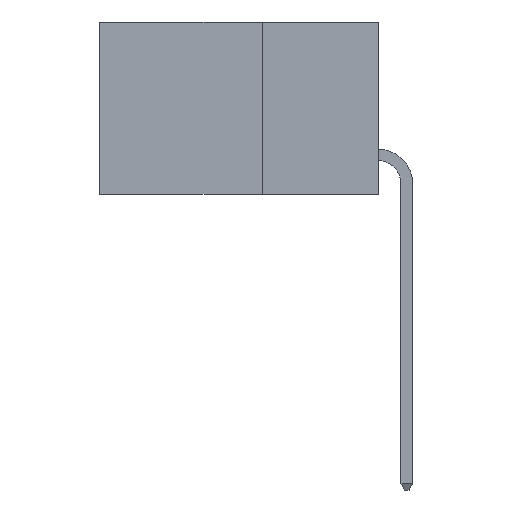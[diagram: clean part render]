
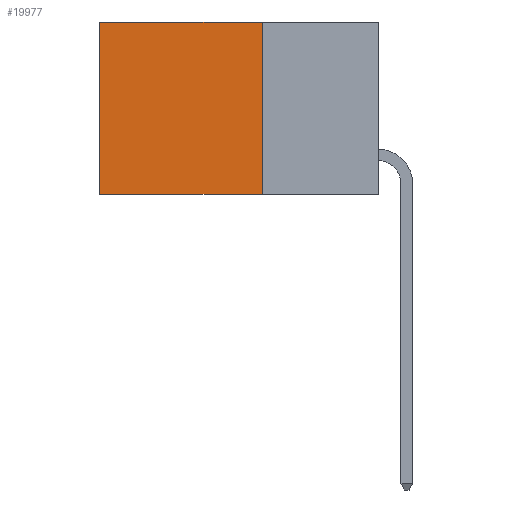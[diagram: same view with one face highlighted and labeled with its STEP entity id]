
A CAD part, left-side view. The second image highlights one B-rep face of the part: STEP entity #19977.
In plain terms, the highlighted planar face has unit normal (-1, 0, 0).
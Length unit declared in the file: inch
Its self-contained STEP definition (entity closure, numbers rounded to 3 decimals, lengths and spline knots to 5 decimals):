
#441 = CARTESIAN_POINT ( 'NONE',  ( 0.2615, 0.6, -0.37 ) ) ;
#476 = DIRECTION ( 'NONE',  ( 0., 0., -1. ) ) ;
#864 = VERTEX_POINT ( 'NONE', #13997 ) ;
#1123 = VECTOR ( 'NONE', #1857, 39.37008 ) ;
#1793 = LINE ( 'NONE', #8405, #6531 ) ;
#1857 = DIRECTION ( 'NONE',  ( 0., 1., 0. ) ) ;
#1906 = EDGE_CURVE ( 'NONE', #5128, #5581, #18871, .T. ) ;
#2567 = VECTOR ( 'NONE', #17411, 39.37008 ) ;
#3395 = VERTEX_POINT ( 'NONE', #441 ) ;
#3829 = VECTOR ( 'NONE', #476, 39.37008 ) ;
#4305 = AXIS2_PLACEMENT_3D ( 'NONE', #18575, #9163, #20146 ) ;
#5128 = VERTEX_POINT ( 'NONE', #12304 ) ;
#5581 = VERTEX_POINT ( 'NONE', #6313 ) ;
#5906 = ORIENTED_EDGE ( 'NONE', *, *, #7297, .F. ) ;
#6313 = CARTESIAN_POINT ( 'NONE',  ( 0.2615, 0.6, 0. ) ) ;
#6531 = VECTOR ( 'NONE', #17853, 39.37008 ) ;
#7297 = EDGE_CURVE ( 'NONE', #864, #3395, #8578, .T. ) ;
#7581 = PLANE ( 'NONE',  #4305 ) ;
#8405 = CARTESIAN_POINT ( 'NONE',  ( 0.2615, 0.25, -0.37 ) ) ;
#8578 = LINE ( 'NONE', #14553, #1123 ) ;
#9163 = DIRECTION ( 'NONE',  ( 1., 0., 0. ) ) ;
#9313 = EDGE_CURVE ( 'NONE', #5128, #864, #1793, .T. ) ;
#9955 = ORIENTED_EDGE ( 'NONE', *, *, #18941, .T. ) ;
#12304 = CARTESIAN_POINT ( 'NONE',  ( 0.2615, 0.25, 0. ) ) ;
#13202 = ORIENTED_EDGE ( 'NONE', *, *, #9313, .F. ) ;
#13216 = EDGE_LOOP ( 'NONE', ( #9955, #5906, #13202, #16206 ) ) ;
#13997 = CARTESIAN_POINT ( 'NONE',  ( 0.2615, 0.25, -0.37 ) ) ;
#14553 = CARTESIAN_POINT ( 'NONE',  ( 0.2615, 0.25, -0.37 ) ) ;
#16206 = ORIENTED_EDGE ( 'NONE', *, *, #1906, .T. ) ;
#16438 = FACE_OUTER_BOUND ( 'NONE', #13216, .T. ) ;
#16460 = LINE ( 'NONE', #17780, #3829 ) ;
#17411 = DIRECTION ( 'NONE',  ( 0., 1., 0. ) ) ;
#17780 = CARTESIAN_POINT ( 'NONE',  ( 0.2615, 0.6, -0.37 ) ) ;
#17853 = DIRECTION ( 'NONE',  ( 0., 0., -1. ) ) ;
#18575 = CARTESIAN_POINT ( 'NONE',  ( 0.2615, 0.25, -0.37 ) ) ;
#18871 = LINE ( 'NONE', #20050, #2567 ) ;
#18941 = EDGE_CURVE ( 'NONE', #5581, #3395, #16460, .T. ) ;
#19977 = ADVANCED_FACE ( 'NONE', ( #16438 ), #7581, .F. ) ;
#20050 = CARTESIAN_POINT ( 'NONE',  ( 0.2615, 0.25, 0. ) ) ;
#20146 = DIRECTION ( 'NONE',  ( 0., 0., -1. ) ) ;
